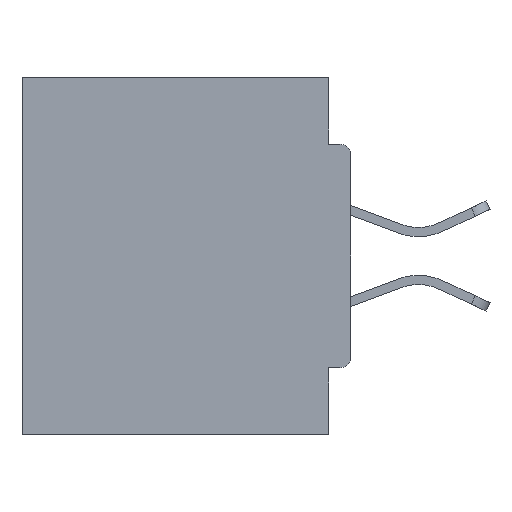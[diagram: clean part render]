
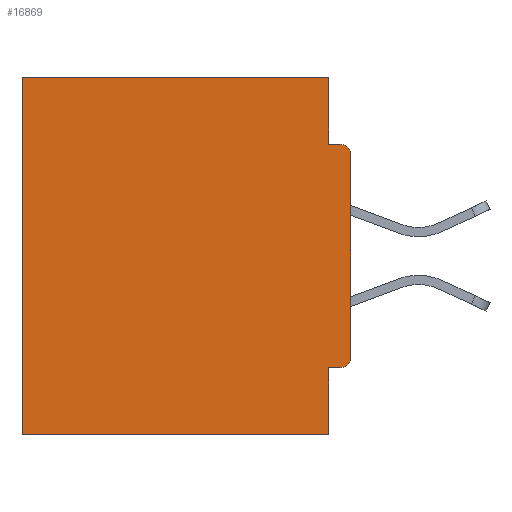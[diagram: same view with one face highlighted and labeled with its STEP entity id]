
A CAD part, left-side view. The second image highlights one B-rep face of the part: STEP entity #16869.
In plain terms, the highlighted planar face has unit normal (-1, 0, 0).
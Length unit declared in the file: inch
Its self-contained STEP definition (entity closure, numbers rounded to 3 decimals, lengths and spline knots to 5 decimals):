
#9 = DIRECTION ( 'NONE',  ( 0., 0., -1. ) ) ;
#146 = EDGE_CURVE ( 'NONE', #2132, #17979, #13370, .T. ) ;
#337 = ORIENTED_EDGE ( 'NONE', *, *, #19248, .T. ) ;
#467 = CARTESIAN_POINT ( 'NONE',  ( 0.298, 0.031, 0. ) ) ;
#521 = CARTESIAN_POINT ( 'NONE',  ( 0.298, 0.46, 0. ) ) ;
#1744 = LINE ( 'NONE', #31977, #12095 ) ;
#2132 = VERTEX_POINT ( 'NONE', #3227 ) ;
#2146 = CARTESIAN_POINT ( 'NONE',  ( 0.298, 0.031, -0.5 ) ) ;
#2672 = VERTEX_POINT ( 'NONE', #6169 ) ;
#2709 = CARTESIAN_POINT ( 'NONE',  ( 0.298, 0.46, -0.5 ) ) ;
#3092 = ORIENTED_EDGE ( 'NONE', *, *, #12566, .T. ) ;
#3227 = CARTESIAN_POINT ( 'NONE',  ( 0.298, 0., -0.1085 ) ) ;
#4023 = CARTESIAN_POINT ( 'NONE',  ( 0.298, 0., 0. ) ) ;
#5169 = VECTOR ( 'NONE', #24928, 39.37008 ) ;
#5616 = CARTESIAN_POINT ( 'NONE',  ( 0.298, 0.031, -0.5 ) ) ;
#6169 = CARTESIAN_POINT ( 'NONE',  ( 0.298, 0.015, -0.4065 ) ) ;
#6190 = EDGE_CURVE ( 'NONE', #2672, #7457, #33433, .T. ) ;
#6318 = PLANE ( 'NONE',  #35478 ) ;
#6525 = EDGE_CURVE ( 'NONE', #12005, #10679, #30366, .T. ) ;
#7232 = VERTEX_POINT ( 'NONE', #9740 ) ;
#7457 = VERTEX_POINT ( 'NONE', #29384 ) ;
#8839 = CARTESIAN_POINT ( 'NONE',  ( 0.298, 0.015, -0.3915 ) ) ;
#9333 = DIRECTION ( 'NONE',  ( 0., 1., 0. ) ) ;
#9583 = LINE ( 'NONE', #2146, #27765 ) ;
#9723 = EDGE_CURVE ( 'NONE', #13345, #17979, #34279, .T. ) ;
#9740 = CARTESIAN_POINT ( 'NONE',  ( 0.298, 0.031, -0.5 ) ) ;
#10358 = ORIENTED_EDGE ( 'NONE', *, *, #9723, .F. ) ;
#10679 = VERTEX_POINT ( 'NONE', #21752 ) ;
#11503 = DIRECTION ( 'NONE',  ( 0., 0., -1. ) ) ;
#12005 = VERTEX_POINT ( 'NONE', #467 ) ;
#12095 = VECTOR ( 'NONE', #24071, 39.37008 ) ;
#12566 = EDGE_CURVE ( 'NONE', #10679, #23442, #28925, .T. ) ;
#12922 = VERTEX_POINT ( 'NONE', #24293 ) ;
#13195 = EDGE_CURVE ( 'NONE', #7232, #23442, #31425, .T. ) ;
#13345 = VERTEX_POINT ( 'NONE', #28233 ) ;
#13370 = CIRCLE ( 'NONE', #18432, 0.015 ) ;
#14096 = CIRCLE ( 'NONE', #24019, 0.015 ) ;
#14111 = DIRECTION ( 'NONE',  ( -1., 0., 0. ) ) ;
#15076 = VECTOR ( 'NONE', #28426, 39.37008 ) ;
#15684 = VECTOR ( 'NONE', #23228, 39.37008 ) ;
#16068 = CARTESIAN_POINT ( 'NONE',  ( 0.298, 0.015, -0.0935 ) ) ;
#16144 = ORIENTED_EDGE ( 'NONE', *, *, #6525, .T. ) ;
#16869 = ADVANCED_FACE ( 'NONE', ( #23333 ), #6318, .F. ) ;
#17979 = VERTEX_POINT ( 'NONE', #16068 ) ;
#18432 = AXIS2_PLACEMENT_3D ( 'NONE', #30665, #14111, #9 ) ;
#19248 = EDGE_CURVE ( 'NONE', #2672, #12922, #14096, .T. ) ;
#19636 = ORIENTED_EDGE ( 'NONE', *, *, #29602, .F. ) ;
#20312 = DIRECTION ( 'NONE',  ( 0., 0., -1. ) ) ;
#21752 = CARTESIAN_POINT ( 'NONE',  ( 0.298, 0.46, 0. ) ) ;
#22336 = DIRECTION ( 'NONE',  ( -1., 0., 0. ) ) ;
#22553 = VECTOR ( 'NONE', #35430, 39.37008 ) ;
#23228 = DIRECTION ( 'NONE',  ( 0., -1., 0. ) ) ;
#23333 = FACE_OUTER_BOUND ( 'NONE', #33107, .T. ) ;
#23442 = VERTEX_POINT ( 'NONE', #2709 ) ;
#24019 = AXIS2_PLACEMENT_3D ( 'NONE', #8839, #22336, #11503 ) ;
#24037 = VECTOR ( 'NONE', #9333, 39.37008 ) ;
#24071 = DIRECTION ( 'NONE',  ( 0., 0., -1. ) ) ;
#24094 = DIRECTION ( 'NONE',  ( 0., 0., -1. ) ) ;
#24293 = CARTESIAN_POINT ( 'NONE',  ( 0.298, 0., -0.3915 ) ) ;
#24547 = ORIENTED_EDGE ( 'NONE', *, *, #146, .T. ) ;
#24928 = DIRECTION ( 'NONE',  ( 0., 0., -1. ) ) ;
#25667 = EDGE_CURVE ( 'NONE', #2132, #12922, #1744, .T. ) ;
#25870 = CARTESIAN_POINT ( 'NONE',  ( 0.298, 0., -0.5 ) ) ;
#26152 = CARTESIAN_POINT ( 'NONE',  ( 0.298, 0., -0.0935 ) ) ;
#27226 = LINE ( 'NONE', #5616, #5169 ) ;
#27765 = VECTOR ( 'NONE', #24094, 39.37008 ) ;
#28233 = CARTESIAN_POINT ( 'NONE',  ( 0.298, 0.031, -0.0935 ) ) ;
#28426 = DIRECTION ( 'NONE',  ( 0., 0., -1. ) ) ;
#28925 = LINE ( 'NONE', #521, #15076 ) ;
#28936 = DIRECTION ( 'NONE',  ( 1., 0., 0. ) ) ;
#29310 = ORIENTED_EDGE ( 'NONE', *, *, #13195, .F. ) ;
#29384 = CARTESIAN_POINT ( 'NONE',  ( 0.298, 0.031, -0.4065 ) ) ;
#29446 = ORIENTED_EDGE ( 'NONE', *, *, #25667, .F. ) ;
#29602 = EDGE_CURVE ( 'NONE', #7457, #7232, #9583, .T. ) ;
#30366 = LINE ( 'NONE', #31967, #35141 ) ;
#30665 = CARTESIAN_POINT ( 'NONE',  ( 0.298, 0.015, -0.1085 ) ) ;
#30877 = EDGE_CURVE ( 'NONE', #12005, #13345, #27226, .T. ) ;
#31425 = LINE ( 'NONE', #25870, #24037 ) ;
#31967 = CARTESIAN_POINT ( 'NONE',  ( 0.298, 0., 0. ) ) ;
#31977 = CARTESIAN_POINT ( 'NONE',  ( 0.298, 0., 0. ) ) ;
#32576 = ORIENTED_EDGE ( 'NONE', *, *, #6190, .F. ) ;
#33107 = EDGE_LOOP ( 'NONE', ( #24547, #10358, #34464, #16144, #3092, #29310, #19636, #32576, #337, #29446 ) ) ;
#33433 = LINE ( 'NONE', #35314, #22553 ) ;
#34279 = LINE ( 'NONE', #26152, #15684 ) ;
#34294 = DIRECTION ( 'NONE',  ( 0., 1., 0. ) ) ;
#34464 = ORIENTED_EDGE ( 'NONE', *, *, #30877, .F. ) ;
#35141 = VECTOR ( 'NONE', #34294, 39.37008 ) ;
#35314 = CARTESIAN_POINT ( 'NONE',  ( 0.298, 0., -0.4065 ) ) ;
#35430 = DIRECTION ( 'NONE',  ( 0., 1., 0. ) ) ;
#35478 = AXIS2_PLACEMENT_3D ( 'NONE', #4023, #28936, #20312 ) ;
